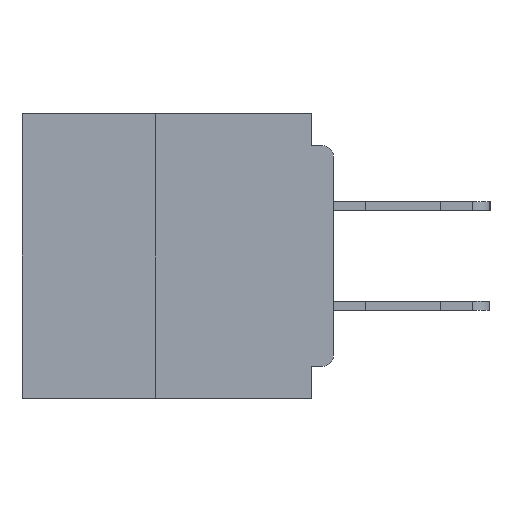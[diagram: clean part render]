
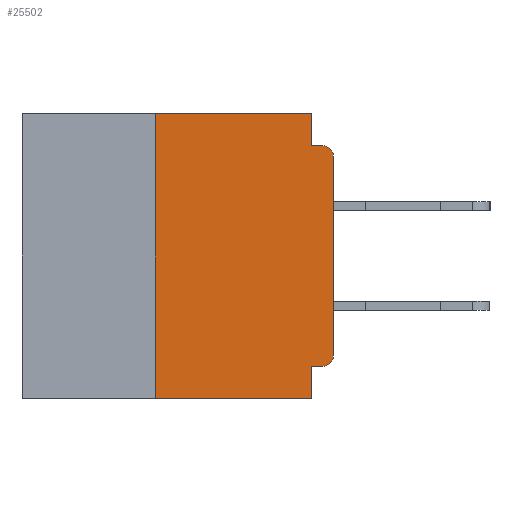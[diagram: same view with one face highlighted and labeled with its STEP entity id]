
A CAD part, left-side view. The second image highlights one B-rep face of the part: STEP entity #25502.
In plain terms, the highlighted planar face has unit normal (-1, 0, 0).
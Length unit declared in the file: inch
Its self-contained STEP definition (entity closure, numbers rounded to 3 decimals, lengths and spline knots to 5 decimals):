
#225 = EDGE_CURVE ( 'NONE', #13798, #50315, #16612, .T. ) ;
#341 = VERTEX_POINT ( 'NONE', #36597 ) ;
#1063 = EDGE_LOOP ( 'NONE', ( #25859, #9843, #37544, #51286, #39887, #19444, #18341, #6437, #4013, #9980 ) ) ;
#2446 = CARTESIAN_POINT ( 'NONE',  ( 0., 0.031, 0. ) ) ;
#2663 = LINE ( 'NONE', #35022, #44177 ) ;
#4013 = ORIENTED_EDGE ( 'NONE', *, *, #6899, .F. ) ;
#4122 = DIRECTION ( 'NONE',  ( 1., 0., 0. ) ) ;
#4779 = VERTEX_POINT ( 'NONE', #6885 ) ;
#6127 = CARTESIAN_POINT ( 'NONE',  ( 0., 0.437, -0.4 ) ) ;
#6437 = ORIENTED_EDGE ( 'NONE', *, *, #38789, .F. ) ;
#6885 = CARTESIAN_POINT ( 'NONE',  ( 0., 0.031, -0.4 ) ) ;
#6899 = EDGE_CURVE ( 'NONE', #17730, #28968, #2663, .T. ) ;
#7048 = DIRECTION ( 'NONE',  ( 0., 1., 0. ) ) ;
#7125 = CARTESIAN_POINT ( 'NONE',  ( 0., 0.015, -0.045 ) ) ;
#8296 = CARTESIAN_POINT ( 'NONE',  ( 0., 0.015, -0.06 ) ) ;
#9402 = VECTOR ( 'NONE', #42150, 39.37008 ) ;
#9843 = ORIENTED_EDGE ( 'NONE', *, *, #10848, .T. ) ;
#9980 = ORIENTED_EDGE ( 'NONE', *, *, #19779, .T. ) ;
#10848 = EDGE_CURVE ( 'NONE', #50315, #35663, #16256, .T. ) ;
#12336 = DIRECTION ( 'NONE',  ( 0., 0., -1. ) ) ;
#12617 = VERTEX_POINT ( 'NONE', #42084 ) ;
#13463 = VECTOR ( 'NONE', #23858, 39.37008 ) ;
#13798 = VERTEX_POINT ( 'NONE', #42160 ) ;
#14064 = CARTESIAN_POINT ( 'NONE',  ( 0., 0., -0.045 ) ) ;
#14248 = CARTESIAN_POINT ( 'NONE',  ( 0., 0., -0.06 ) ) ;
#15059 = CARTESIAN_POINT ( 'NONE',  ( 0., 0.015, -0.34 ) ) ;
#15174 = EDGE_CURVE ( 'NONE', #12617, #35663, #50769, .T. ) ;
#15632 = VECTOR ( 'NONE', #49455, 39.37008 ) ;
#16256 = CIRCLE ( 'NONE', #44619, 0.015 ) ;
#16612 = LINE ( 'NONE', #50281, #46040 ) ;
#17730 = VERTEX_POINT ( 'NONE', #38092 ) ;
#18341 = ORIENTED_EDGE ( 'NONE', *, *, #24619, .T. ) ;
#18346 = DIRECTION ( 'NONE',  ( 0., -1., 0. ) ) ;
#18841 = DIRECTION ( 'NONE',  ( 0., 0., -1. ) ) ;
#19166 = DIRECTION ( 'NONE',  ( 0., 0., -1. ) ) ;
#19187 = CIRCLE ( 'NONE', #24483, 0.015 ) ;
#19444 = ORIENTED_EDGE ( 'NONE', *, *, #47264, .F. ) ;
#19779 = EDGE_CURVE ( 'NONE', #17730, #13798, #19187, .T. ) ;
#19824 = CARTESIAN_POINT ( 'NONE',  ( 0., 0.25, -0.4 ) ) ;
#20381 = VECTOR ( 'NONE', #18841, 39.37008 ) ;
#21960 = VECTOR ( 'NONE', #42904, 39.37008 ) ;
#23858 = DIRECTION ( 'NONE',  ( 0., 0., 1. ) ) ;
#24039 = VERTEX_POINT ( 'NONE', #2446 ) ;
#24483 = AXIS2_PLACEMENT_3D ( 'NONE', #15059, #43110, #19166 ) ;
#24619 = EDGE_CURVE ( 'NONE', #45927, #4779, #46806, .T. ) ;
#25502 = ADVANCED_FACE ( 'NONE', ( #44910 ), #40185, .F. ) ;
#25859 = ORIENTED_EDGE ( 'NONE', *, *, #225, .T. ) ;
#26849 = CARTESIAN_POINT ( 'NONE',  ( 0., 0.031, 0. ) ) ;
#27598 = CARTESIAN_POINT ( 'NONE',  ( 0., 0.031, -0.355 ) ) ;
#28251 = CARTESIAN_POINT ( 'NONE',  ( 0., 0.437, 0. ) ) ;
#28968 = VERTEX_POINT ( 'NONE', #27598 ) ;
#32291 = DIRECTION ( 'NONE',  ( 0., 0., -1. ) ) ;
#32457 = CARTESIAN_POINT ( 'NONE',  ( 0., 0.25, -0.4 ) ) ;
#32612 = LINE ( 'NONE', #34872, #21960 ) ;
#33054 = AXIS2_PLACEMENT_3D ( 'NONE', #28251, #4122, #32291 ) ;
#34872 = CARTESIAN_POINT ( 'NONE',  ( 0., 0.437, 0. ) ) ;
#35022 = CARTESIAN_POINT ( 'NONE',  ( 0., 0., -0.355 ) ) ;
#35586 = EDGE_CURVE ( 'NONE', #24039, #12617, #42892, .T. ) ;
#35663 = VERTEX_POINT ( 'NONE', #7125 ) ;
#36443 = DIRECTION ( 'NONE',  ( -1., 0., 0. ) ) ;
#36597 = CARTESIAN_POINT ( 'NONE',  ( 0., 0.25, 0. ) ) ;
#37544 = ORIENTED_EDGE ( 'NONE', *, *, #15174, .F. ) ;
#38092 = CARTESIAN_POINT ( 'NONE',  ( 0., 0.015, -0.355 ) ) ;
#38789 = EDGE_CURVE ( 'NONE', #28968, #4779, #46335, .T. ) ;
#39887 = ORIENTED_EDGE ( 'NONE', *, *, #49079, .F. ) ;
#40185 = PLANE ( 'NONE',  #33054 ) ;
#42084 = CARTESIAN_POINT ( 'NONE',  ( 0., 0.031, -0.045 ) ) ;
#42150 = DIRECTION ( 'NONE',  ( 0., -1., 0. ) ) ;
#42160 = CARTESIAN_POINT ( 'NONE',  ( 0., 0., -0.34 ) ) ;
#42892 = LINE ( 'NONE', #26849, #20381 ) ;
#42904 = DIRECTION ( 'NONE',  ( 0., -1., 0. ) ) ;
#43110 = DIRECTION ( 'NONE',  ( -1., 0., 0. ) ) ;
#44177 = VECTOR ( 'NONE', #7048, 39.37008 ) ;
#44619 = AXIS2_PLACEMENT_3D ( 'NONE', #8296, #36443, #12336 ) ;
#44910 = FACE_OUTER_BOUND ( 'NONE', #1063, .T. ) ;
#45114 = CARTESIAN_POINT ( 'NONE',  ( 0., 0.031, -0.4 ) ) ;
#45466 = LINE ( 'NONE', #19824, #13463 ) ;
#45534 = VECTOR ( 'NONE', #18346, 39.37008 ) ;
#45927 = VERTEX_POINT ( 'NONE', #32457 ) ;
#46040 = VECTOR ( 'NONE', #48658, 39.37008 ) ;
#46335 = LINE ( 'NONE', #45114, #15632 ) ;
#46806 = LINE ( 'NONE', #6127, #45534 ) ;
#47264 = EDGE_CURVE ( 'NONE', #45927, #341, #45466, .T. ) ;
#48658 = DIRECTION ( 'NONE',  ( 0., 0., 1. ) ) ;
#49079 = EDGE_CURVE ( 'NONE', #341, #24039, #32612, .T. ) ;
#49455 = DIRECTION ( 'NONE',  ( 0., 0., -1. ) ) ;
#50281 = CARTESIAN_POINT ( 'NONE',  ( 0., 0., 0. ) ) ;
#50315 = VERTEX_POINT ( 'NONE', #14248 ) ;
#50769 = LINE ( 'NONE', #14064, #9402 ) ;
#51286 = ORIENTED_EDGE ( 'NONE', *, *, #35586, .F. ) ;
